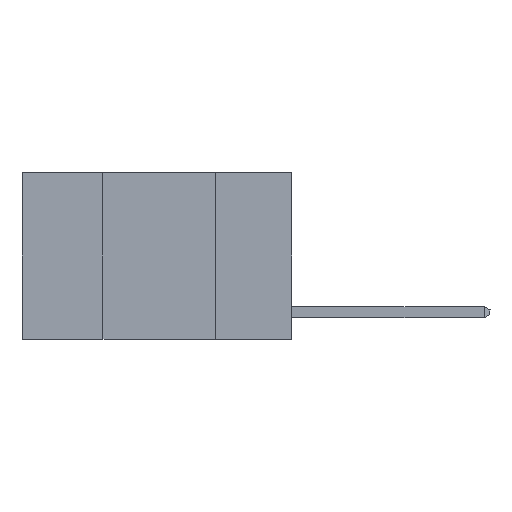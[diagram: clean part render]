
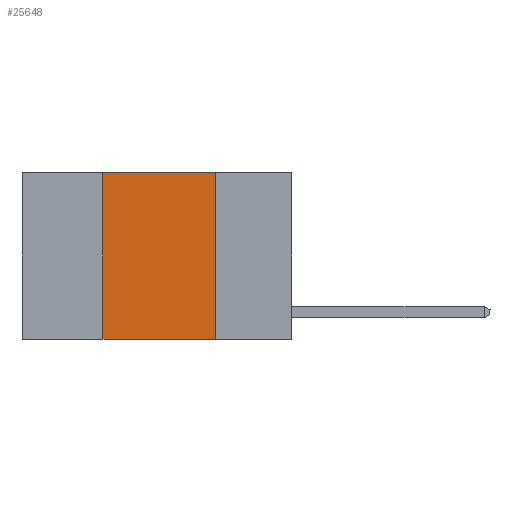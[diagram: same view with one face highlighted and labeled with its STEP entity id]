
A CAD part, left-side view. The second image highlights one B-rep face of the part: STEP entity #25648.
In plain terms, the highlighted planar face has unit normal (-1, 0, 0).
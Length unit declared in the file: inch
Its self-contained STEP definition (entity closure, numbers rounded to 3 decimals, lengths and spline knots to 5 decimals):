
#54 = ORIENTED_EDGE ( 'NONE', *, *, #12292, .F. ) ;
#144 = VECTOR ( 'NONE', #13899, 39.37008 ) ;
#245 = DIRECTION ( 'NONE',  ( 0., 0., -1. ) ) ;
#409 = LINE ( 'NONE', #7453, #144 ) ;
#2483 = VERTEX_POINT ( 'NONE', #14256 ) ;
#4807 = VECTOR ( 'NONE', #21449, 39.37008 ) ;
#5144 = EDGE_CURVE ( 'NONE', #20325, #10093, #15303, .T. ) ;
#5517 = ORIENTED_EDGE ( 'NONE', *, *, #5144, .T. ) ;
#6460 = DIRECTION ( 'NONE',  ( 0., 0., -1. ) ) ;
#7453 = CARTESIAN_POINT ( 'NONE',  ( 0., 0.42, 0. ) ) ;
#7709 = VECTOR ( 'NONE', #245, 39.37008 ) ;
#7730 = CARTESIAN_POINT ( 'NONE',  ( 0., 0.17, 0. ) ) ;
#8380 = EDGE_CURVE ( 'NONE', #2483, #19796, #23704, .T. ) ;
#9367 = EDGE_CURVE ( 'NONE', #20325, #2483, #409, .T. ) ;
#9461 = CARTESIAN_POINT ( 'NONE',  ( 0., 0.17, 0. ) ) ;
#10093 = VERTEX_POINT ( 'NONE', #14590 ) ;
#10874 = DIRECTION ( 'NONE',  ( 0., -1., 0. ) ) ;
#11503 = CARTESIAN_POINT ( 'NONE',  ( 0., 0.42, -0.37 ) ) ;
#12292 = EDGE_CURVE ( 'NONE', #19796, #10093, #13864, .T. ) ;
#12414 = CARTESIAN_POINT ( 'NONE',  ( 0., 0.6, 0. ) ) ;
#12537 = ORIENTED_EDGE ( 'NONE', *, *, #9367, .F. ) ;
#13463 = DIRECTION ( 'NONE',  ( 1., 0., 0. ) ) ;
#13864 = LINE ( 'NONE', #9461, #7709 ) ;
#13899 = DIRECTION ( 'NONE',  ( 0., 0., 1. ) ) ;
#14256 = CARTESIAN_POINT ( 'NONE',  ( 0., 0.42, 0. ) ) ;
#14590 = CARTESIAN_POINT ( 'NONE',  ( 0., 0.17, -0.37 ) ) ;
#15303 = LINE ( 'NONE', #24353, #17479 ) ;
#16180 = EDGE_LOOP ( 'NONE', ( #54, #20803, #12537, #5517 ) ) ;
#17479 = VECTOR ( 'NONE', #10874, 39.37008 ) ;
#17595 = AXIS2_PLACEMENT_3D ( 'NONE', #26792, #13463, #6460 ) ;
#19796 = VERTEX_POINT ( 'NONE', #7730 ) ;
#19999 = FACE_OUTER_BOUND ( 'NONE', #16180, .T. ) ;
#20325 = VERTEX_POINT ( 'NONE', #11503 ) ;
#20803 = ORIENTED_EDGE ( 'NONE', *, *, #8380, .F. ) ;
#21449 = DIRECTION ( 'NONE',  ( 0., -1., 0. ) ) ;
#23704 = LINE ( 'NONE', #12414, #4807 ) ;
#24353 = CARTESIAN_POINT ( 'NONE',  ( 0., 0.6, -0.37 ) ) ;
#25648 = ADVANCED_FACE ( 'NONE', ( #19999 ), #28978, .F. ) ;
#26792 = CARTESIAN_POINT ( 'NONE',  ( 0., 0.6, 0. ) ) ;
#28978 = PLANE ( 'NONE',  #17595 ) ;
